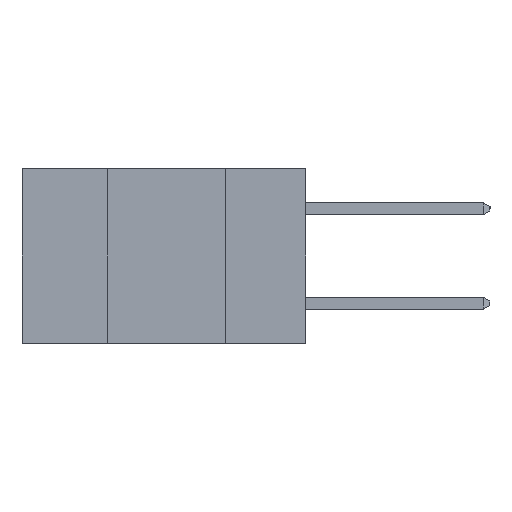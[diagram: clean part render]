
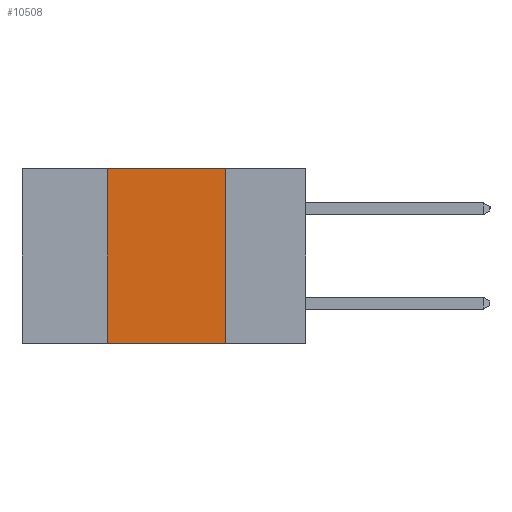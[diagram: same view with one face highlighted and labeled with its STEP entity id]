
A CAD part, left-side view. The second image highlights one B-rep face of the part: STEP entity #10508.
In plain terms, the highlighted planar face has unit normal (-1, 0, 0).
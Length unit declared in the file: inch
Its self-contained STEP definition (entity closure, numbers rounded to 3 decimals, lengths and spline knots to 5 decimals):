
#429 = DIRECTION ( 'NONE',  ( 0., 0., -1. ) ) ;
#1575 = CARTESIAN_POINT ( 'NONE',  ( 0., 0.6, -0.37 ) ) ;
#1691 = DIRECTION ( 'NONE',  ( 0., -1., 0. ) ) ;
#1708 = CARTESIAN_POINT ( 'NONE',  ( 0., 0.17, 0. ) ) ;
#2006 = ORIENTED_EDGE ( 'NONE', *, *, #6167, .F. ) ;
#2244 = DIRECTION ( 'NONE',  ( 1., 0., 0. ) ) ;
#2418 = CARTESIAN_POINT ( 'NONE',  ( 0., 0.17, -0.37 ) ) ;
#2611 = EDGE_CURVE ( 'NONE', #4245, #4243, #4215, .T. ) ;
#3286 = LINE ( 'NONE', #1575, #7438 ) ;
#3366 = VERTEX_POINT ( 'NONE', #9755 ) ;
#3469 = CARTESIAN_POINT ( 'NONE',  ( 0., 0.42, 0. ) ) ;
#3930 = EDGE_LOOP ( 'NONE', ( #9054, #6056, #2006, #6049 ) ) ;
#4046 = CARTESIAN_POINT ( 'NONE',  ( 0., 0.6, 0. ) ) ;
#4215 = LINE ( 'NONE', #4046, #7717 ) ;
#4243 = VERTEX_POINT ( 'NONE', #1708 ) ;
#4245 = VERTEX_POINT ( 'NONE', #3469 ) ;
#5328 = DIRECTION ( 'NONE',  ( 0., 0., 1. ) ) ;
#6049 = ORIENTED_EDGE ( 'NONE', *, *, #10073, .T. ) ;
#6056 = ORIENTED_EDGE ( 'NONE', *, *, #2611, .F. ) ;
#6167 = EDGE_CURVE ( 'NONE', #6486, #4245, #7048, .T. ) ;
#6419 = CARTESIAN_POINT ( 'NONE',  ( 0., 0.42, -0.37 ) ) ;
#6486 = VERTEX_POINT ( 'NONE', #7081 ) ;
#6833 = DIRECTION ( 'NONE',  ( 0., -1., 0. ) ) ;
#6859 = LINE ( 'NONE', #2418, #8548 ) ;
#7048 = LINE ( 'NONE', #6419, #10495 ) ;
#7081 = CARTESIAN_POINT ( 'NONE',  ( 0., 0.42, -0.37 ) ) ;
#7438 = VECTOR ( 'NONE', #1691, 39.37008 ) ;
#7717 = VECTOR ( 'NONE', #6833, 39.37008 ) ;
#8277 = PLANE ( 'NONE',  #8722 ) ;
#8548 = VECTOR ( 'NONE', #10334, 39.37008 ) ;
#8722 = AXIS2_PLACEMENT_3D ( 'NONE', #10054, #2244, #429 ) ;
#9054 = ORIENTED_EDGE ( 'NONE', *, *, #10610, .F. ) ;
#9755 = CARTESIAN_POINT ( 'NONE',  ( 0., 0.17, -0.37 ) ) ;
#10054 = CARTESIAN_POINT ( 'NONE',  ( 0., 0.6, 0. ) ) ;
#10073 = EDGE_CURVE ( 'NONE', #6486, #3366, #3286, .T. ) ;
#10334 = DIRECTION ( 'NONE',  ( 0., 0., -1. ) ) ;
#10495 = VECTOR ( 'NONE', #5328, 39.37008 ) ;
#10508 = ADVANCED_FACE ( 'NONE', ( #10917 ), #8277, .F. ) ;
#10610 = EDGE_CURVE ( 'NONE', #4243, #3366, #6859, .T. ) ;
#10917 = FACE_OUTER_BOUND ( 'NONE', #3930, .T. ) ;
